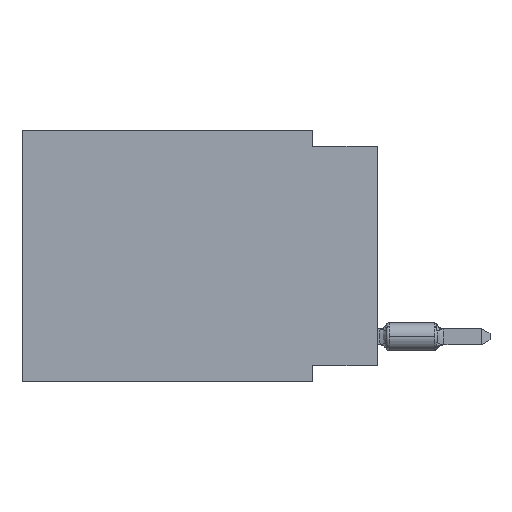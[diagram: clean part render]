
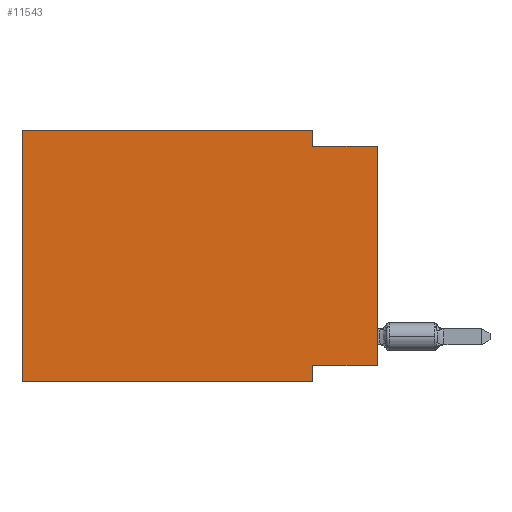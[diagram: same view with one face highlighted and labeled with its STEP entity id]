
A CAD part, left-side view. The second image highlights one B-rep face of the part: STEP entity #11543.
In plain terms, the highlighted planar face has unit normal (-1, 0, 0).
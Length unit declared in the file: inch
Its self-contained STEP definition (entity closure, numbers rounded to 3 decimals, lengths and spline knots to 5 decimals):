
#30 = DIRECTION ( 'NONE',  ( 0., 0., -1. ) ) ;
#222 = VECTOR ( 'NONE', #11603, 39.37008 ) ;
#1414 = EDGE_CURVE ( 'NONE', #1689, #23299, #16586, .T. ) ;
#1513 = FACE_OUTER_BOUND ( 'NONE', #9276, .T. ) ;
#1689 = VERTEX_POINT ( 'NONE', #4480 ) ;
#2135 = LINE ( 'NONE', #13074, #27982 ) ;
#2468 = EDGE_CURVE ( 'NONE', #22809, #9879, #20447, .T. ) ;
#3408 = DIRECTION ( 'NONE',  ( 0., -1., 0. ) ) ;
#3771 = LINE ( 'NONE', #18973, #13594 ) ;
#4278 = EDGE_CURVE ( 'NONE', #19006, #27178, #26007, .T. ) ;
#4480 = CARTESIAN_POINT ( 'NONE',  ( 0., 0., -0.365 ) ) ;
#4481 = CARTESIAN_POINT ( 'NONE',  ( 0., 0., -0.025 ) ) ;
#5424 = CARTESIAN_POINT ( 'NONE',  ( 0., 0.1, -0.39 ) ) ;
#5843 = CARTESIAN_POINT ( 'NONE',  ( 0., 0.1, -0.365 ) ) ;
#6749 = VECTOR ( 'NONE', #3408, 39.37008 ) ;
#7204 = EDGE_CURVE ( 'NONE', #27178, #22809, #3771, .T. ) ;
#7445 = CARTESIAN_POINT ( 'NONE',  ( 0., 0.1, 0. ) ) ;
#8251 = ORIENTED_EDGE ( 'NONE', *, *, #25235, .T. ) ;
#8862 = CARTESIAN_POINT ( 'NONE',  ( 0., 0., -0.025 ) ) ;
#9276 = EDGE_LOOP ( 'NONE', ( #28957, #15132, #9703, #20341, #25231, #8251, #18843, #27323 ) ) ;
#9357 = LINE ( 'NONE', #4481, #19424 ) ;
#9571 = CARTESIAN_POINT ( 'NONE',  ( 0., 0.1, -0.025 ) ) ;
#9703 = ORIENTED_EDGE ( 'NONE', *, *, #2468, .F. ) ;
#9879 = VERTEX_POINT ( 'NONE', #9571 ) ;
#10141 = DIRECTION ( 'NONE',  ( 0., -1., 0. ) ) ;
#10679 = EDGE_CURVE ( 'NONE', #9879, #15960, #9357, .T. ) ;
#10721 = DIRECTION ( 'NONE',  ( 0., 0., 1. ) ) ;
#11543 = ADVANCED_FACE ( 'NONE', ( #1513 ), #22780, .F. ) ;
#11603 = DIRECTION ( 'NONE',  ( 0., 0., -1. ) ) ;
#13074 = CARTESIAN_POINT ( 'NONE',  ( 0., 0., 0. ) ) ;
#13491 = DIRECTION ( 'NONE',  ( 0., -1., 0. ) ) ;
#13594 = VECTOR ( 'NONE', #10141, 39.37008 ) ;
#13769 = DIRECTION ( 'NONE',  ( 1., 0., 0. ) ) ;
#13913 = CARTESIAN_POINT ( 'NONE',  ( 0., 0.55, 0. ) ) ;
#14474 = CARTESIAN_POINT ( 'NONE',  ( 0., 0.55, -0.39 ) ) ;
#14957 = VERTEX_POINT ( 'NONE', #20212 ) ;
#15132 = ORIENTED_EDGE ( 'NONE', *, *, #10679, .F. ) ;
#15952 = VECTOR ( 'NONE', #17025, 39.37008 ) ;
#15960 = VERTEX_POINT ( 'NONE', #8862 ) ;
#16586 = LINE ( 'NONE', #17179, #15952 ) ;
#17025 = DIRECTION ( 'NONE',  ( 0., 1., 0. ) ) ;
#17179 = CARTESIAN_POINT ( 'NONE',  ( 0., 0., -0.365 ) ) ;
#18001 = EDGE_CURVE ( 'NONE', #1689, #15960, #2135, .T. ) ;
#18151 = CARTESIAN_POINT ( 'NONE',  ( 0., 0.1, 0. ) ) ;
#18751 = CARTESIAN_POINT ( 'NONE',  ( 0., 0.55, 0. ) ) ;
#18843 = ORIENTED_EDGE ( 'NONE', *, *, #25633, .F. ) ;
#18973 = CARTESIAN_POINT ( 'NONE',  ( 0., 0.55, 0. ) ) ;
#19006 = VERTEX_POINT ( 'NONE', #19589 ) ;
#19424 = VECTOR ( 'NONE', #13491, 39.37008 ) ;
#19589 = CARTESIAN_POINT ( 'NONE',  ( 0., 0.55, -0.39 ) ) ;
#20212 = CARTESIAN_POINT ( 'NONE',  ( 0., 0.1, -0.39 ) ) ;
#20341 = ORIENTED_EDGE ( 'NONE', *, *, #7204, .F. ) ;
#20447 = LINE ( 'NONE', #7445, #222 ) ;
#21407 = DIRECTION ( 'NONE',  ( 0., 0., 1. ) ) ;
#22780 = PLANE ( 'NONE',  #26968 ) ;
#22809 = VERTEX_POINT ( 'NONE', #18151 ) ;
#23299 = VERTEX_POINT ( 'NONE', #5843 ) ;
#23649 = LINE ( 'NONE', #14474, #6749 ) ;
#24426 = CARTESIAN_POINT ( 'NONE',  ( 0., 0.55, 0. ) ) ;
#25231 = ORIENTED_EDGE ( 'NONE', *, *, #4278, .F. ) ;
#25235 = EDGE_CURVE ( 'NONE', #19006, #14957, #23649, .T. ) ;
#25633 = EDGE_CURVE ( 'NONE', #23299, #14957, #25658, .T. ) ;
#25658 = LINE ( 'NONE', #5424, #28931 ) ;
#25810 = DIRECTION ( 'NONE',  ( 0., 0., -1. ) ) ;
#26007 = LINE ( 'NONE', #18751, #28719 ) ;
#26968 = AXIS2_PLACEMENT_3D ( 'NONE', #13913, #13769, #30 ) ;
#27178 = VERTEX_POINT ( 'NONE', #24426 ) ;
#27323 = ORIENTED_EDGE ( 'NONE', *, *, #1414, .F. ) ;
#27982 = VECTOR ( 'NONE', #10721, 39.37008 ) ;
#28719 = VECTOR ( 'NONE', #21407, 39.37008 ) ;
#28931 = VECTOR ( 'NONE', #25810, 39.37008 ) ;
#28957 = ORIENTED_EDGE ( 'NONE', *, *, #18001, .T. ) ;
